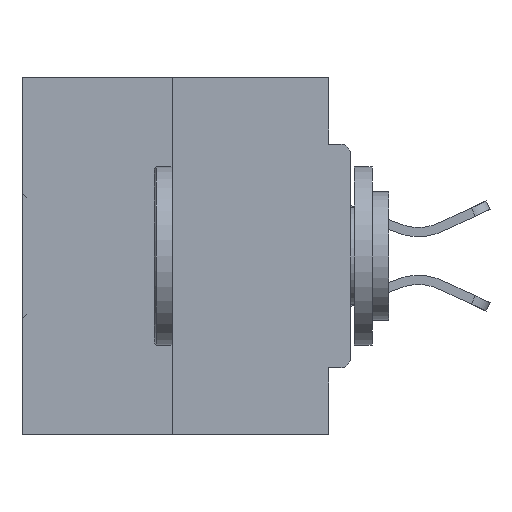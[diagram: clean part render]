
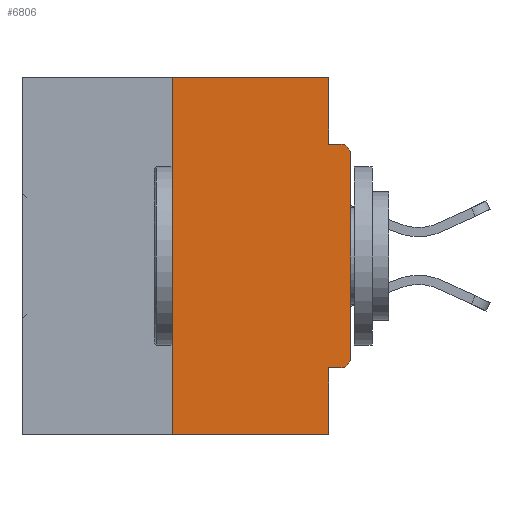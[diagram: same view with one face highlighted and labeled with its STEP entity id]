
A CAD part, left-side view. The second image highlights one B-rep face of the part: STEP entity #6806.
In plain terms, the highlighted planar face has unit normal (-1, 0, 0).
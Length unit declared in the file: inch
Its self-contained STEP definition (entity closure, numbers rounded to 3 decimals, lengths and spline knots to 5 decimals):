
#167 = DIRECTION ( 'NONE',  ( 0., 1., 0. ) ) ;
#321 = CARTESIAN_POINT ( 'NONE',  ( 0., 0.46, 0. ) ) ;
#661 = AXIS2_PLACEMENT_3D ( 'NONE', #24779, #10494, #3256 ) ;
#1246 = CIRCLE ( 'NONE', #5990, 0.015 ) ;
#3153 = EDGE_CURVE ( 'NONE', #34204, #40148, #10835, .T. ) ;
#3256 = DIRECTION ( 'NONE',  ( 0., 0., -1. ) ) ;
#3263 = EDGE_CURVE ( 'NONE', #28334, #14774, #20931, .T. ) ;
#3971 = ORIENTED_EDGE ( 'NONE', *, *, #37495, .T. ) ;
#5264 = DIRECTION ( 'NONE',  ( -1., 0., 0. ) ) ;
#5565 = CARTESIAN_POINT ( 'NONE',  ( 0., 0.015, -0.4065 ) ) ;
#5740 = DIRECTION ( 'NONE',  ( 0., 0., -1. ) ) ;
#5990 = AXIS2_PLACEMENT_3D ( 'NONE', #9348, #5264, #5740 ) ;
#6238 = DIRECTION ( 'NONE',  ( 0., 0., -1. ) ) ;
#6279 = AXIS2_PLACEMENT_3D ( 'NONE', #33270, #37574, #15955 ) ;
#6722 = DIRECTION ( 'NONE',  ( 0., 0., 1. ) ) ;
#6806 = ADVANCED_FACE ( 'NONE', ( #37806 ), #14083, .F. ) ;
#7360 = CARTESIAN_POINT ( 'NONE',  ( 0., 0.25, -0.5 ) ) ;
#8057 = LINE ( 'NONE', #42274, #19892 ) ;
#8890 = CARTESIAN_POINT ( 'NONE',  ( 0., 0.031, -0.0935 ) ) ;
#9066 = ORIENTED_EDGE ( 'NONE', *, *, #3263, .T. ) ;
#9085 = EDGE_CURVE ( 'NONE', #27282, #11680, #39283, .T. ) ;
#9348 = CARTESIAN_POINT ( 'NONE',  ( 0., 0.015, -0.3915 ) ) ;
#9776 = EDGE_CURVE ( 'NONE', #13345, #22767, #10992, .T. ) ;
#10494 = DIRECTION ( 'NONE',  ( 1., 0., 0. ) ) ;
#10778 = VECTOR ( 'NONE', #6238, 39.37008 ) ;
#10835 = LINE ( 'NONE', #36844, #22052 ) ;
#10976 = CARTESIAN_POINT ( 'NONE',  ( 0., 0.031, 0. ) ) ;
#10992 = LINE ( 'NONE', #321, #19411 ) ;
#11405 = ORIENTED_EDGE ( 'NONE', *, *, #12495, .T. ) ;
#11541 = ORIENTED_EDGE ( 'NONE', *, *, #13668, .F. ) ;
#11680 = VERTEX_POINT ( 'NONE', #16804 ) ;
#11974 = VECTOR ( 'NONE', #6722, 39.37008 ) ;
#12495 = EDGE_CURVE ( 'NONE', #14774, #40148, #44798, .T. ) ;
#13125 = ORIENTED_EDGE ( 'NONE', *, *, #32820, .F. ) ;
#13345 = VERTEX_POINT ( 'NONE', #29664 ) ;
#13668 = EDGE_CURVE ( 'NONE', #18722, #11680, #29333, .T. ) ;
#14083 = PLANE ( 'NONE',  #661 ) ;
#14774 = VERTEX_POINT ( 'NONE', #30184 ) ;
#15955 = DIRECTION ( 'NONE',  ( 0., 0., -1. ) ) ;
#16747 = CARTESIAN_POINT ( 'NONE',  ( 0., 0.031, -0.5 ) ) ;
#16804 = CARTESIAN_POINT ( 'NONE',  ( 0., 0.031, -0.5 ) ) ;
#18722 = VERTEX_POINT ( 'NONE', #45462 ) ;
#18730 = CARTESIAN_POINT ( 'NONE',  ( 0., 0.031, 0. ) ) ;
#19411 = VECTOR ( 'NONE', #21854, 39.37008 ) ;
#19892 = VECTOR ( 'NONE', #30353, 39.37008 ) ;
#20156 = ORIENTED_EDGE ( 'NONE', *, *, #9085, .T. ) ;
#20931 = LINE ( 'NONE', #24767, #11974 ) ;
#21640 = ORIENTED_EDGE ( 'NONE', *, *, #29101, .F. ) ;
#21854 = DIRECTION ( 'NONE',  ( 0., -1., 0. ) ) ;
#22017 = CARTESIAN_POINT ( 'NONE',  ( 0., 0., -0.4065 ) ) ;
#22052 = VECTOR ( 'NONE', #37319, 39.37008 ) ;
#22767 = VERTEX_POINT ( 'NONE', #18730 ) ;
#23034 = VERTEX_POINT ( 'NONE', #5565 ) ;
#24767 = CARTESIAN_POINT ( 'NONE',  ( 0., 0., 0. ) ) ;
#24779 = CARTESIAN_POINT ( 'NONE',  ( 0., 0.46, 0. ) ) ;
#26665 = ORIENTED_EDGE ( 'NONE', *, *, #3153, .F. ) ;
#26835 = VECTOR ( 'NONE', #167, 39.37008 ) ;
#27220 = LINE ( 'NONE', #10976, #30601 ) ;
#27282 = VERTEX_POINT ( 'NONE', #7360 ) ;
#27917 = CARTESIAN_POINT ( 'NONE',  ( 0., 0., -0.3915 ) ) ;
#28334 = VERTEX_POINT ( 'NONE', #27917 ) ;
#28431 = DIRECTION ( 'NONE',  ( 0., 0., -1. ) ) ;
#29021 = DIRECTION ( 'NONE',  ( 0., -1., 0. ) ) ;
#29101 = EDGE_CURVE ( 'NONE', #23034, #18722, #36466, .T. ) ;
#29333 = LINE ( 'NONE', #16747, #10778 ) ;
#29664 = CARTESIAN_POINT ( 'NONE',  ( 0., 0.25, 0. ) ) ;
#30184 = CARTESIAN_POINT ( 'NONE',  ( 0., 0., -0.1085 ) ) ;
#30353 = DIRECTION ( 'NONE',  ( 0., 0., 1. ) ) ;
#30601 = VECTOR ( 'NONE', #28431, 39.37008 ) ;
#30732 = VECTOR ( 'NONE', #29021, 39.37008 ) ;
#31276 = CARTESIAN_POINT ( 'NONE',  ( 0., 0.015, -0.0935 ) ) ;
#32820 = EDGE_CURVE ( 'NONE', #22767, #34204, #27220, .T. ) ;
#33270 = CARTESIAN_POINT ( 'NONE',  ( 0., 0.015, -0.1085 ) ) ;
#34204 = VERTEX_POINT ( 'NONE', #8890 ) ;
#36466 = LINE ( 'NONE', #22017, #26835 ) ;
#36844 = CARTESIAN_POINT ( 'NONE',  ( 0., 0., -0.0935 ) ) ;
#37160 = EDGE_LOOP ( 'NONE', ( #45424, #41154, #20156, #11541, #21640, #3971, #9066, #11405, #26665, #13125 ) ) ;
#37319 = DIRECTION ( 'NONE',  ( 0., -1., 0. ) ) ;
#37495 = EDGE_CURVE ( 'NONE', #23034, #28334, #1246, .T. ) ;
#37574 = DIRECTION ( 'NONE',  ( -1., 0., 0. ) ) ;
#37806 = FACE_OUTER_BOUND ( 'NONE', #37160, .T. ) ;
#39283 = LINE ( 'NONE', #40107, #30732 ) ;
#40107 = CARTESIAN_POINT ( 'NONE',  ( 0., 0.46, -0.5 ) ) ;
#40148 = VERTEX_POINT ( 'NONE', #31276 ) ;
#41154 = ORIENTED_EDGE ( 'NONE', *, *, #42430, .F. ) ;
#42274 = CARTESIAN_POINT ( 'NONE',  ( 0., 0.25, 0. ) ) ;
#42430 = EDGE_CURVE ( 'NONE', #27282, #13345, #8057, .T. ) ;
#44798 = CIRCLE ( 'NONE', #6279, 0.015 ) ;
#45424 = ORIENTED_EDGE ( 'NONE', *, *, #9776, .F. ) ;
#45462 = CARTESIAN_POINT ( 'NONE',  ( 0., 0.031, -0.4065 ) ) ;
